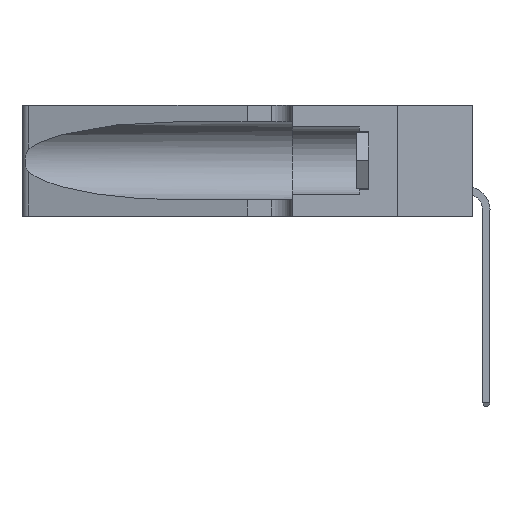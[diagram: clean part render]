
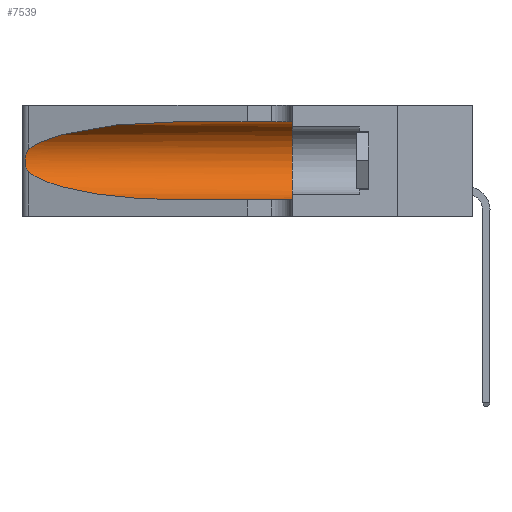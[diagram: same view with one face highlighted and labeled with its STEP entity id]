
A CAD part, left-side view. The second image highlights one B-rep face of the part: STEP entity #7539.
In plain terms, the highlighted cylindrical face has radius 3.308 mm (diameter 6.617 mm), a partial arc.
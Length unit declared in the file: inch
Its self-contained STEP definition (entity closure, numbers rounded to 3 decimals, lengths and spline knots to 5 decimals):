
#587 = CARTESIAN_POINT ( 'NONE',  ( 0.1305, 0.35, 0.31525 ) ) ;
#1845 = DIRECTION ( 'NONE',  ( 0., -1., 0. ) ) ;
#2060 = CARTESIAN_POINT ( 'NONE',  ( 0.1305, 1.61858, 0.185 ) ) ;
#2616 = ORIENTED_EDGE ( 'NONE', *, *, #16931, .F. ) ;
#3202 = FACE_OUTER_BOUND ( 'NONE', #16504, .T. ) ;
#3245 = CARTESIAN_POINT ( 'NONE',  ( 0.1305, 0.35, 0.185 ) ) ;
#3722 = VERTEX_POINT ( 'NONE', #5235 ) ;
#3886 = ORIENTED_EDGE ( 'NONE', *, *, #4359, .T. ) ;
#3893 = CARTESIAN_POINT ( 'NONE',  ( 0.2373, 1.15595, 0.28018 ) ) ;
#3975 = VECTOR ( 'NONE', #4150, 39.37008 ) ;
#4111 = ORIENTED_EDGE ( 'NONE', *, *, #11375, .T. ) ;
#4150 = DIRECTION ( 'NONE',  ( 0., -1., 0. ) ) ;
#4343 = VERTEX_POINT ( 'NONE', #17873 ) ;
#4359 = EDGE_CURVE ( 'NONE', #15429, #11919, #7362, .T. ) ;
#4378 = VERTEX_POINT ( 'NONE', #9317 ) ;
#4597 = CARTESIAN_POINT ( 'NONE',  ( 0.1305, 1.61858, 0.31525 ) ) ;
#4982 = CARTESIAN_POINT ( 'NONE',  ( 0.26075, 1.23896, 0.19203 ) ) ;
#5210 = EDGE_CURVE ( 'NONE', #4343, #3722, #14359, .T. ) ;
#5235 = CARTESIAN_POINT ( 'NONE',  ( 0.1305, 0.35, 0.05475 ) ) ;
#5428 = CARTESIAN_POINT ( 'NONE',  ( 0.18966, 0.96281, 0.05475 ) ) ;
#6076 = EDGE_CURVE ( 'NONE', #11919, #4378, #16433, .T. ) ;
#6283 = CARTESIAN_POINT ( 'NONE',  ( 0.26075, 1.23896, 0.178 ) ) ;
#6469 = DIRECTION ( 'NONE',  ( 0., -1., 0. ) ) ;
#6473 = CARTESIAN_POINT ( 'NONE',  ( 0.18966, 0.96281, 0.31525 ) ) ;
#7039 = EDGE_CURVE ( 'NONE', #17745, #3722, #17848, .T. ) ;
#7362 =( BOUNDED_CURVE ( )  B_SPLINE_CURVE ( 3, ( #13779, #6473, #3893, #13714 ),
 .UNSPECIFIED., .F., .F. ) 
 B_SPLINE_CURVE_WITH_KNOTS ( ( 4, 4 ),
 ( 1.5708, 2.84003 ),
 .UNSPECIFIED. ) 
 CURVE ( )  GEOMETRIC_REPRESENTATION_ITEM ( )  RATIONAL_B_SPLINE_CURVE ( ( 1., 0.87, 0.87, 1. ) ) 
 REPRESENTATION_ITEM ( '' )  );
#7539 = ADVANCED_FACE ( 'NONE', ( #3202 ), #16480, .F. ) ;
#7628 = ORIENTED_EDGE ( 'NONE', *, *, #7039, .F. ) ;
#8505 = CARTESIAN_POINT ( 'NONE',  ( 0.25487, 1.22718, 0.14631 ) ) ;
#8636 = CARTESIAN_POINT ( 'NONE',  ( 0.25854, 1.2359, 0.20912 ) ) ;
#9195 = DIRECTION ( 'NONE',  ( 0., 0., -1. ) ) ;
#9317 = CARTESIAN_POINT ( 'NONE',  ( 0.25487, 1.22718, 0.14631 ) ) ;
#10045 = CARTESIAN_POINT ( 'NONE',  ( 0.25555, 1.22993, 0.14849 ) ) ;
#10219 = LINE ( 'NONE', #4597, #10888 ) ;
#10888 = VECTOR ( 'NONE', #1845, 39.37008 ) ;
#11138 = CARTESIAN_POINT ( 'NONE',  ( 0.25487, 1.22718, 0.22369 ) ) ;
#11375 = EDGE_CURVE ( 'NONE', #4378, #4343, #14741, .T. ) ;
#11783 = DIRECTION ( 'NONE',  ( 0., 1., 0. ) ) ;
#11919 = VERTEX_POINT ( 'NONE', #14513 ) ;
#12226 = CARTESIAN_POINT ( 'NONE',  ( 0.25639, 1.23186, 0.15144 ) ) ;
#12419 = CARTESIAN_POINT ( 'NONE',  ( 0.25487, 1.22718, 0.14631 ) ) ;
#12551 = CARTESIAN_POINT ( 'NONE',  ( 0.25555, 1.22994, 0.2215 ) ) ;
#12680 = CARTESIAN_POINT ( 'NONE',  ( 0.1305, 1.61858, 0.05475 ) ) ;
#13269 = CARTESIAN_POINT ( 'NONE',  ( 0.26017, 1.23833, 0.17102 ) ) ;
#13714 = CARTESIAN_POINT ( 'NONE',  ( 0.25487, 1.22718, 0.22369 ) ) ;
#13779 = CARTESIAN_POINT ( 'NONE',  ( 0.1305, 0.72297, 0.31525 ) ) ;
#14359 = LINE ( 'NONE', #12680, #3975 ) ;
#14513 = CARTESIAN_POINT ( 'NONE',  ( 0.25487, 1.22718, 0.22369 ) ) ;
#14684 = CARTESIAN_POINT ( 'NONE',  ( 0.1305, 0.72297, 0.31525 ) ) ;
#14706 = CARTESIAN_POINT ( 'NONE',  ( 0.25856, 1.23593, 0.16098 ) ) ;
#14741 =( BOUNDED_CURVE ( )  B_SPLINE_CURVE ( 3, ( #12419, #16804, #5428, #15196 ),
 .UNSPECIFIED., .F., .T. ) 
 B_SPLINE_CURVE_WITH_KNOTS ( ( 4, 4 ),
 ( 3.44316, 4.71239 ),
 .UNSPECIFIED. ) 
 CURVE ( )  GEOMETRIC_REPRESENTATION_ITEM ( )  RATIONAL_B_SPLINE_CURVE ( ( 1., 0.87, 0.87, 1. ) ) 
 REPRESENTATION_ITEM ( '' )  );
#14928 = DIRECTION ( 'NONE',  ( 0., 0., 1. ) ) ;
#14993 = AXIS2_PLACEMENT_3D ( 'NONE', #3245, #11783, #14928 ) ;
#15122 = ORIENTED_EDGE ( 'NONE', *, *, #6076, .T. ) ;
#15196 = CARTESIAN_POINT ( 'NONE',  ( 0.1305, 0.72297, 0.05475 ) ) ;
#15429 = VERTEX_POINT ( 'NONE', #14684 ) ;
#15438 = CARTESIAN_POINT ( 'NONE',  ( 0.25639, 1.23184, 0.21858 ) ) ;
#16118 = CARTESIAN_POINT ( 'NONE',  ( 0.25789, 1.23486, 0.15765 ) ) ;
#16433 = B_SPLINE_CURVE_WITH_KNOTS ( 'NONE', 3,
 ( #11138, #12551, #15438, #16880, #8636, #17492, #4982, #6283, #13269, #14706, #16118, #12226, #10045, #8505 ),
 .UNSPECIFIED., .F., .F.,
 ( 4, 2, 2, 2, 2, 2, 4 ),
 ( 0., 0.00027, 0.00053, 0.00107, 0.0016, 0.00187, 0.00214 ),
 .UNSPECIFIED. ) ;
#16480 = CYLINDRICAL_SURFACE ( 'NONE', #16672, 0.13025 ) ;
#16504 = EDGE_LOOP ( 'NONE', ( #3886, #15122, #4111, #17048, #7628, #2616 ) ) ;
#16672 = AXIS2_PLACEMENT_3D ( 'NONE', #2060, #6469, #9195 ) ;
#16804 = CARTESIAN_POINT ( 'NONE',  ( 0.2373, 1.15595, 0.08982 ) ) ;
#16880 = CARTESIAN_POINT ( 'NONE',  ( 0.25787, 1.23484, 0.2124 ) ) ;
#16931 = EDGE_CURVE ( 'NONE', #15429, #17745, #10219, .T. ) ;
#17048 = ORIENTED_EDGE ( 'NONE', *, *, #5210, .T. ) ;
#17492 = CARTESIAN_POINT ( 'NONE',  ( 0.26018, 1.23835, 0.19895 ) ) ;
#17745 = VERTEX_POINT ( 'NONE', #587 ) ;
#17848 = CIRCLE ( 'NONE', #14993, 0.13025 ) ;
#17873 = CARTESIAN_POINT ( 'NONE',  ( 0.1305, 0.72297, 0.05475 ) ) ;
